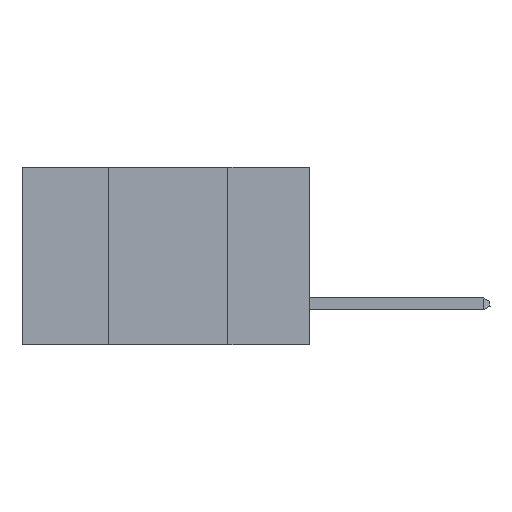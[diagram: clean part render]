
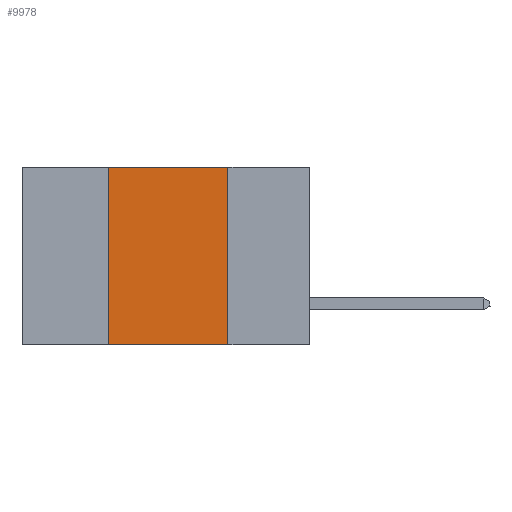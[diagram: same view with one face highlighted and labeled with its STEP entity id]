
A CAD part, left-side view. The second image highlights one B-rep face of the part: STEP entity #9978.
In plain terms, the highlighted planar face has unit normal (-1, 0, 0).
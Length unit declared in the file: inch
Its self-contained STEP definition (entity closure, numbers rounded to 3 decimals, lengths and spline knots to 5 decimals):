
#954 = LINE ( 'NONE', #9612, #10123 ) ;
#959 = CARTESIAN_POINT ( 'NONE',  ( 0., 0.42, -0.37 ) ) ;
#999 = ORIENTED_EDGE ( 'NONE', *, *, #10758, .F. ) ;
#1057 = VERTEX_POINT ( 'NONE', #3270 ) ;
#1531 = ORIENTED_EDGE ( 'NONE', *, *, #5817, .F. ) ;
#2323 = VECTOR ( 'NONE', #10942, 39.37008 ) ;
#2462 = VECTOR ( 'NONE', #5075, 39.37008 ) ;
#3269 = LINE ( 'NONE', #4145, #11456 ) ;
#3270 = CARTESIAN_POINT ( 'NONE',  ( 0., 0.17, 0. ) ) ;
#3459 = FACE_OUTER_BOUND ( 'NONE', #5336, .T. ) ;
#3524 = PLANE ( 'NONE',  #6095 ) ;
#3534 = VERTEX_POINT ( 'NONE', #6861 ) ;
#4145 = CARTESIAN_POINT ( 'NONE',  ( 0., 0.17, 0. ) ) ;
#4739 = VERTEX_POINT ( 'NONE', #9444 ) ;
#5075 = DIRECTION ( 'NONE',  ( 0., -1., 0. ) ) ;
#5156 = VERTEX_POINT ( 'NONE', #959 ) ;
#5336 = EDGE_LOOP ( 'NONE', ( #10495, #1531, #999, #6985 ) ) ;
#5498 = EDGE_CURVE ( 'NONE', #1057, #3534, #3269, .T. ) ;
#5817 = EDGE_CURVE ( 'NONE', #4739, #1057, #9322, .T. ) ;
#6095 = AXIS2_PLACEMENT_3D ( 'NONE', #7286, #11179, #11362 ) ;
#6861 = CARTESIAN_POINT ( 'NONE',  ( 0., 0.17, -0.37 ) ) ;
#6985 = ORIENTED_EDGE ( 'NONE', *, *, #10178, .T. ) ;
#7286 = CARTESIAN_POINT ( 'NONE',  ( 0., 0.6, 0. ) ) ;
#7966 = DIRECTION ( 'NONE',  ( 0., 0., -1. ) ) ;
#9322 = LINE ( 'NONE', #11200, #2462 ) ;
#9444 = CARTESIAN_POINT ( 'NONE',  ( 0., 0.42, 0. ) ) ;
#9612 = CARTESIAN_POINT ( 'NONE',  ( 0., 0.6, -0.37 ) ) ;
#9978 = ADVANCED_FACE ( 'NONE', ( #3459 ), #3524, .F. ) ;
#10123 = VECTOR ( 'NONE', #11489, 39.37008 ) ;
#10178 = EDGE_CURVE ( 'NONE', #5156, #3534, #954, .T. ) ;
#10495 = ORIENTED_EDGE ( 'NONE', *, *, #5498, .F. ) ;
#10758 = EDGE_CURVE ( 'NONE', #5156, #4739, #11833, .T. ) ;
#10942 = DIRECTION ( 'NONE',  ( 0., 0., 1. ) ) ;
#11179 = DIRECTION ( 'NONE',  ( 1., 0., 0. ) ) ;
#11200 = CARTESIAN_POINT ( 'NONE',  ( 0., 0.6, 0. ) ) ;
#11362 = DIRECTION ( 'NONE',  ( 0., 0., -1. ) ) ;
#11456 = VECTOR ( 'NONE', #7966, 39.37008 ) ;
#11489 = DIRECTION ( 'NONE',  ( 0., -1., 0. ) ) ;
#11833 = LINE ( 'NONE', #11899, #2323 ) ;
#11899 = CARTESIAN_POINT ( 'NONE',  ( 0., 0.42, 0. ) ) ;
